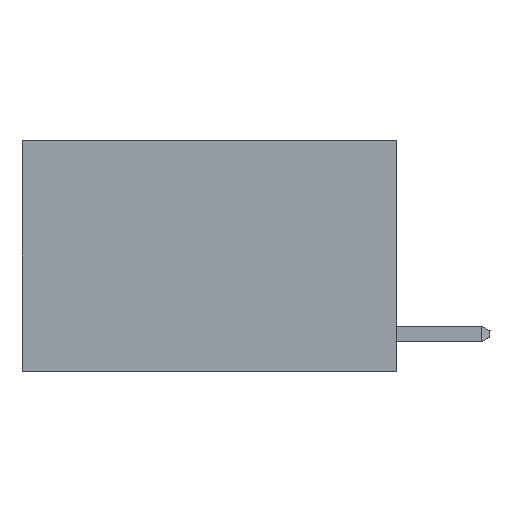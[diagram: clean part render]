
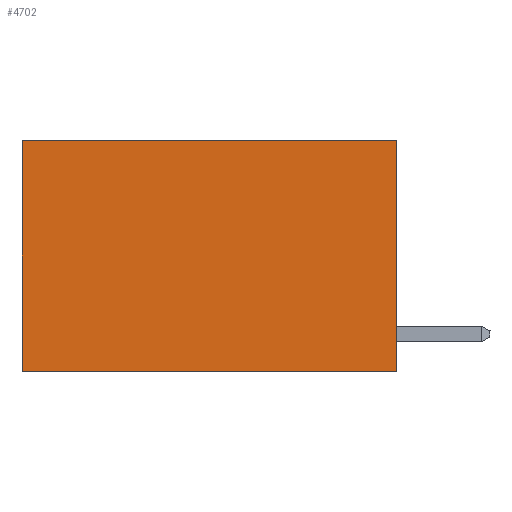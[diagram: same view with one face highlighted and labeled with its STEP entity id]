
A CAD part, left-side view. The second image highlights one B-rep face of the part: STEP entity #4702.
In plain terms, the highlighted planar face has unit normal (-1, 0, 0).
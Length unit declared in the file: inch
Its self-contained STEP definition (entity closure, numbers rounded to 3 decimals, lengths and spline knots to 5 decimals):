
#2442 = LINE ( 'NONE', #14968, #21424 ) ;
#2843 = VECTOR ( 'NONE', #5213, 39.37008 ) ;
#4069 = LINE ( 'NONE', #18094, #2843 ) ;
#4231 = EDGE_LOOP ( 'NONE', ( #13764, #6495, #16655, #17820 ) ) ;
#4702 = ADVANCED_FACE ( 'NONE', ( #23104 ), #5036, .F. ) ;
#5036 = PLANE ( 'NONE',  #13043 ) ;
#5213 = DIRECTION ( 'NONE',  ( 0., 1., 0. ) ) ;
#6495 = ORIENTED_EDGE ( 'NONE', *, *, #9026, .F. ) ;
#6863 = DIRECTION ( 'NONE',  ( 0., 0., -1. ) ) ;
#6988 = DIRECTION ( 'NONE',  ( 0., 0., -1. ) ) ;
#7408 = CARTESIAN_POINT ( 'NONE',  ( 0.2625, 0., 0. ) ) ;
#8361 = EDGE_CURVE ( 'NONE', #19398, #9553, #19654, .T. ) ;
#8379 = CARTESIAN_POINT ( 'NONE',  ( 0.2625, 0.6, 0. ) ) ;
#9026 = EDGE_CURVE ( 'NONE', #9553, #16728, #4069, .T. ) ;
#9553 = VERTEX_POINT ( 'NONE', #15984 ) ;
#9652 = LINE ( 'NONE', #8379, #18654 ) ;
#10271 = DIRECTION ( 'NONE',  ( 0., 0., -1. ) ) ;
#12507 = CARTESIAN_POINT ( 'NONE',  ( 0.2625, 0., 0. ) ) ;
#13043 = AXIS2_PLACEMENT_3D ( 'NONE', #12507, #17931, #6988 ) ;
#13764 = ORIENTED_EDGE ( 'NONE', *, *, #19760, .T. ) ;
#14968 = CARTESIAN_POINT ( 'NONE',  ( 0.2625, 0., 0. ) ) ;
#15984 = CARTESIAN_POINT ( 'NONE',  ( 0.2625, 0., -0.37 ) ) ;
#16655 = ORIENTED_EDGE ( 'NONE', *, *, #8361, .F. ) ;
#16728 = VERTEX_POINT ( 'NONE', #20083 ) ;
#17607 = EDGE_CURVE ( 'NONE', #19398, #20761, #2442, .T. ) ;
#17820 = ORIENTED_EDGE ( 'NONE', *, *, #17607, .T. ) ;
#17931 = DIRECTION ( 'NONE',  ( 1., 0., 0. ) ) ;
#18094 = CARTESIAN_POINT ( 'NONE',  ( 0.2625, 0., -0.37 ) ) ;
#18654 = VECTOR ( 'NONE', #10271, 39.37008 ) ;
#19104 = VECTOR ( 'NONE', #6863, 39.37008 ) ;
#19398 = VERTEX_POINT ( 'NONE', #7408 ) ;
#19654 = LINE ( 'NONE', #21284, #19104 ) ;
#19760 = EDGE_CURVE ( 'NONE', #20761, #16728, #9652, .T. ) ;
#20083 = CARTESIAN_POINT ( 'NONE',  ( 0.2625, 0.6, -0.37 ) ) ;
#20088 = CARTESIAN_POINT ( 'NONE',  ( 0.2625, 0.6, 0. ) ) ;
#20761 = VERTEX_POINT ( 'NONE', #20088 ) ;
#21284 = CARTESIAN_POINT ( 'NONE',  ( 0.2625, 0., 0. ) ) ;
#21424 = VECTOR ( 'NONE', #22067, 39.37008 ) ;
#22067 = DIRECTION ( 'NONE',  ( 0., 1., 0. ) ) ;
#23104 = FACE_OUTER_BOUND ( 'NONE', #4231, .T. ) ;
